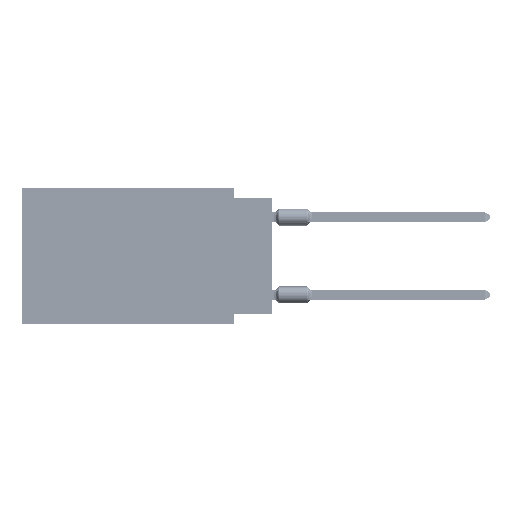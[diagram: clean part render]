
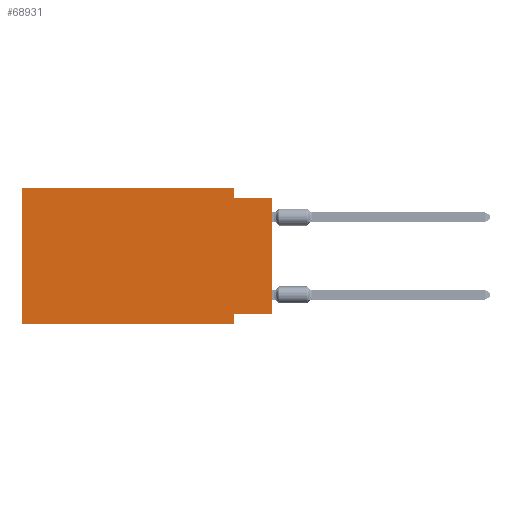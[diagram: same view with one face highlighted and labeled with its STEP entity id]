
A CAD part, left-side view. The second image highlights one B-rep face of the part: STEP entity #68931.
In plain terms, the highlighted planar face has unit normal (-1, 0, 0).
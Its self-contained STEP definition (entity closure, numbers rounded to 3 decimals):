
#554 = VERTEX_POINT ( 'NONE', #41392 ) ;
#3456 = DIRECTION ( 'NONE',  ( 0., -1., 0. ) ) ;
#5023 = VECTOR ( 'NONE', #89435, 1000. ) ;
#5366 = VECTOR ( 'NONE', #45706, 1000. ) ;
#6028 = CARTESIAN_POINT ( 'NONE',  ( 0., 2.54, 0. ) ) ;
#6774 = VERTEX_POINT ( 'NONE', #43921 ) ;
#8706 = ORIENTED_EDGE ( 'NONE', *, *, #48557, .F. ) ;
#11227 = ORIENTED_EDGE ( 'NONE', *, *, #59275, .F. ) ;
#13875 = LINE ( 'NONE', #6028, #5023 ) ;
#14321 = CARTESIAN_POINT ( 'NONE',  ( 0., 0., -0.635 ) ) ;
#15751 = DIRECTION ( 'NONE',  ( 0., 1., 0. ) ) ;
#16187 = CARTESIAN_POINT ( 'NONE',  ( 0., 2.54, -8.89 ) ) ;
#16587 = VERTEX_POINT ( 'NONE', #25196 ) ;
#21330 = CARTESIAN_POINT ( 'NONE',  ( 0., 0., 0. ) ) ;
#21681 = VECTOR ( 'NONE', #93676, 1000. ) ;
#23187 = ORIENTED_EDGE ( 'NONE', *, *, #23294, .T. ) ;
#23294 = EDGE_CURVE ( 'NONE', #6774, #61409, #58599, .T. ) ;
#25196 = CARTESIAN_POINT ( 'NONE',  ( 0., 2.54, -0.635 ) ) ;
#26522 = CARTESIAN_POINT ( 'NONE',  ( 0., 16.383, -8.89 ) ) ;
#28190 = CARTESIAN_POINT ( 'NONE',  ( 0., 2.54, 0. ) ) ;
#29522 = CARTESIAN_POINT ( 'NONE',  ( 0., 16.383, 0. ) ) ;
#31538 = CARTESIAN_POINT ( 'NONE',  ( 0., 2.54, -8.255 ) ) ;
#32739 = EDGE_CURVE ( 'NONE', #6774, #53836, #44727, .T. ) ;
#33347 = CARTESIAN_POINT ( 'NONE',  ( 0., 16.383, 0. ) ) ;
#34205 = CARTESIAN_POINT ( 'NONE',  ( 0., 16.383, 0. ) ) ;
#35280 = LINE ( 'NONE', #33347, #21681 ) ;
#35638 = VECTOR ( 'NONE', #15751, 1000. ) ;
#36107 = EDGE_CURVE ( 'NONE', #53836, #44744, #44686, .T. ) ;
#36255 = VERTEX_POINT ( 'NONE', #71106 ) ;
#36556 = EDGE_LOOP ( 'NONE', ( #23187, #79745, #73380, #8706, #11227, #70734, #53839, #95339 ) ) ;
#41093 = DIRECTION ( 'NONE',  ( 0., 0., -1. ) ) ;
#41392 = CARTESIAN_POINT ( 'NONE',  ( 0., 16.383, -8.89 ) ) ;
#42667 = VECTOR ( 'NONE', #94465, 1000. ) ;
#43921 = CARTESIAN_POINT ( 'NONE',  ( 0., 0., -8.255 ) ) ;
#44686 = LINE ( 'NONE', #16187, #48659 ) ;
#44727 = LINE ( 'NONE', #83446, #35638 ) ;
#44744 = VERTEX_POINT ( 'NONE', #60369 ) ;
#45706 = DIRECTION ( 'NONE',  ( 0., -1., 0. ) ) ;
#47485 = DIRECTION ( 'NONE',  ( 1., 0., 0. ) ) ;
#47969 = FACE_OUTER_BOUND ( 'NONE', #36556, .T. ) ;
#48557 = EDGE_CURVE ( 'NONE', #36255, #70732, #35280, .T. ) ;
#48659 = VECTOR ( 'NONE', #76039, 1000. ) ;
#53047 = LINE ( 'NONE', #14321, #5366 ) ;
#53836 = VERTEX_POINT ( 'NONE', #31538 ) ;
#53839 = ORIENTED_EDGE ( 'NONE', *, *, #36107, .F. ) ;
#57016 = VECTOR ( 'NONE', #3456, 1000. ) ;
#58582 = CARTESIAN_POINT ( 'NONE',  ( 0., 0., -0.635 ) ) ;
#58599 = LINE ( 'NONE', #21330, #42667 ) ;
#59275 = EDGE_CURVE ( 'NONE', #554, #36255, #95271, .T. ) ;
#59960 = EDGE_CURVE ( 'NONE', #16587, #61409, #53047, .T. ) ;
#60369 = CARTESIAN_POINT ( 'NONE',  ( 0., 2.54, -8.89 ) ) ;
#61409 = VERTEX_POINT ( 'NONE', #58582 ) ;
#66195 = EDGE_CURVE ( 'NONE', #70732, #16587, #13875, .T. ) ;
#68931 = ADVANCED_FACE ( 'NONE', ( #47969 ), #92128, .F. ) ;
#70732 = VERTEX_POINT ( 'NONE', #28190 ) ;
#70734 = ORIENTED_EDGE ( 'NONE', *, *, #83653, .T. ) ;
#71106 = CARTESIAN_POINT ( 'NONE',  ( 0., 16.383, 0. ) ) ;
#72709 = DIRECTION ( 'NONE',  ( 0., 0., 1. ) ) ;
#73380 = ORIENTED_EDGE ( 'NONE', *, *, #66195, .F. ) ;
#74145 = AXIS2_PLACEMENT_3D ( 'NONE', #34205, #47485, #41093 ) ;
#75292 = VECTOR ( 'NONE', #72709, 1000. ) ;
#76039 = DIRECTION ( 'NONE',  ( 0., 0., -1. ) ) ;
#78993 = LINE ( 'NONE', #26522, #57016 ) ;
#79745 = ORIENTED_EDGE ( 'NONE', *, *, #59960, .F. ) ;
#83446 = CARTESIAN_POINT ( 'NONE',  ( 0., 0., -8.255 ) ) ;
#83653 = EDGE_CURVE ( 'NONE', #554, #44744, #78993, .T. ) ;
#89435 = DIRECTION ( 'NONE',  ( 0., 0., -1. ) ) ;
#92128 = PLANE ( 'NONE',  #74145 ) ;
#93676 = DIRECTION ( 'NONE',  ( 0., -1., 0. ) ) ;
#94465 = DIRECTION ( 'NONE',  ( 0., 0., 1. ) ) ;
#95271 = LINE ( 'NONE', #29522, #75292 ) ;
#95339 = ORIENTED_EDGE ( 'NONE', *, *, #32739, .F. ) ;
